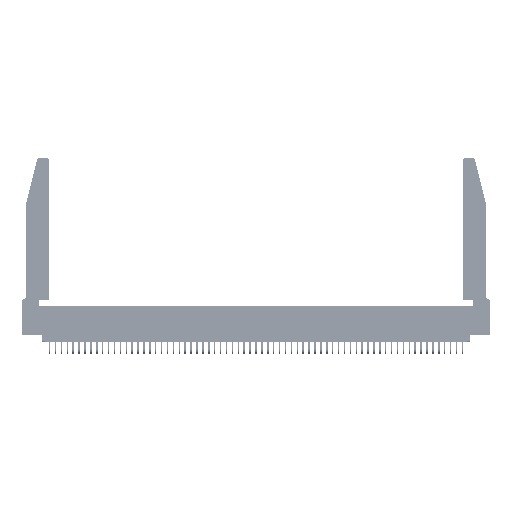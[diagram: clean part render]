
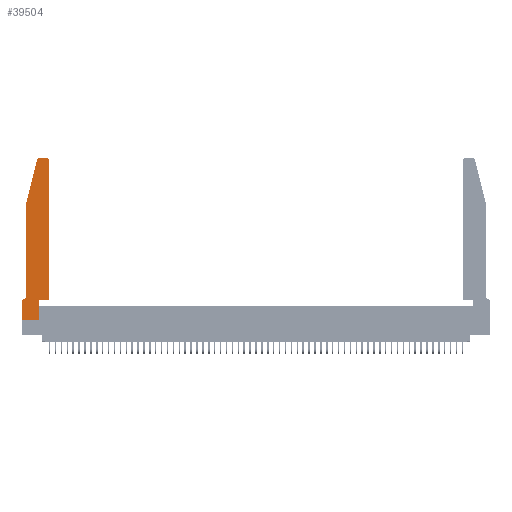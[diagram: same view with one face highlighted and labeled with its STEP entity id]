
A CAD part, top view. The second image highlights one B-rep face of the part: STEP entity #39504.
In plain terms, the highlighted planar face has unit normal (0, 0, 1).
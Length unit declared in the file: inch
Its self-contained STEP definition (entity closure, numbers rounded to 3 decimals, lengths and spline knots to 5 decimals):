
#1034 = VERTEX_POINT ( 'NONE', #20914 ) ;
#1150 = ORIENTED_EDGE ( 'NONE', *, *, #9812, .T. ) ;
#1171 = ORIENTED_EDGE ( 'NONE', *, *, #28467, .T. ) ;
#1255 = DIRECTION ( 'NONE',  ( 0., 0., 1. ) ) ;
#1803 = CARTESIAN_POINT ( 'NONE',  ( 0.25487, 2.72718, 0.37 ) ) ;
#3108 = ORIENTED_EDGE ( 'NONE', *, *, #34720, .T. ) ;
#3602 = VECTOR ( 'NONE', #41435, 39.37008 ) ;
#4488 = VECTOR ( 'NONE', #5732, 39.37008 ) ;
#5732 = DIRECTION ( 'NONE',  ( 0., -1., 0. ) ) ;
#5873 = VERTEX_POINT ( 'NONE', #36605 ) ;
#6295 = LINE ( 'NONE', #46896, #16879 ) ;
#6789 = CARTESIAN_POINT ( 'NONE',  ( 0.2865, 0., 0.37 ) ) ;
#7139 = DIRECTION ( 'NONE',  ( 0., 0., 1. ) ) ;
#7203 = VERTEX_POINT ( 'NONE', #6789 ) ;
#7731 = EDGE_LOOP ( 'NONE', ( #19353, #58043, #13046, #40859, #8081, #19368, #31691, #1150, #57109, #48052, #3108, #1171 ) ) ;
#8081 = ORIENTED_EDGE ( 'NONE', *, *, #39236, .T. ) ;
#9375 = DIRECTION ( 'NONE',  ( 0., 1., 0. ) ) ;
#9408 = VECTOR ( 'NONE', #23605, 39.37008 ) ;
#9812 = EDGE_CURVE ( 'NONE', #35734, #7203, #21348, .T. ) ;
#10364 = EDGE_CURVE ( 'NONE', #39100, #34004, #17067, .T. ) ;
#10908 = EDGE_CURVE ( 'NONE', #15181, #21581, #35340, .T. ) ;
#13046 = ORIENTED_EDGE ( 'NONE', *, *, #24477, .T. ) ;
#13069 = EDGE_CURVE ( 'NONE', #51149, #5873, #43283, .T. ) ;
#13524 = CARTESIAN_POINT ( 'NONE',  ( 0.284, 2.75, 0.37 ) ) ;
#15181 = VERTEX_POINT ( 'NONE', #21804 ) ;
#15740 = CARTESIAN_POINT ( 'NONE',  ( 0.4205, 2.72, 0.37 ) ) ;
#15949 = CARTESIAN_POINT ( 'NONE',  ( 0.2605, 2.75, 0.37 ) ) ;
#16007 = LINE ( 'NONE', #26669, #39957 ) ;
#16879 = VECTOR ( 'NONE', #33489, 39.37008 ) ;
#17067 = CIRCLE ( 'NONE', #20418, 0.03 ) ;
#17629 = DIRECTION ( 'NONE',  ( -0.239, -0.971, 0. ) ) ;
#19092 = CARTESIAN_POINT ( 'NONE',  ( 0., 0., 0.37 ) ) ;
#19340 = VECTOR ( 'NONE', #57221, 39.37008 ) ;
#19353 = ORIENTED_EDGE ( 'NONE', *, *, #34781, .T. ) ;
#19368 = ORIENTED_EDGE ( 'NONE', *, *, #13069, .T. ) ;
#20258 = DIRECTION ( 'NONE',  ( 1., 0., 0. ) ) ;
#20418 = AXIS2_PLACEMENT_3D ( 'NONE', #28280, #1255, #32839 ) ;
#20914 = CARTESIAN_POINT ( 'NONE',  ( 0.2865, 0.35, 0.37 ) ) ;
#21348 = LINE ( 'NONE', #19092, #9408 ) ;
#21581 = VERTEX_POINT ( 'NONE', #56674 ) ;
#21804 = CARTESIAN_POINT ( 'NONE',  ( 0.0755, 2., 0.37 ) ) ;
#21832 = DIRECTION ( 'NONE',  ( 1., 0., 0. ) ) ;
#22284 = VERTEX_POINT ( 'NONE', #38533 ) ;
#23109 = VECTOR ( 'NONE', #21832, 39.37008 ) ;
#23528 = DIRECTION ( 'NONE',  ( 0., 0., -1. ) ) ;
#23605 = DIRECTION ( 'NONE',  ( 1., 0., 0. ) ) ;
#24477 = EDGE_CURVE ( 'NONE', #34004, #15181, #16007, .T. ) ;
#24735 = AXIS2_PLACEMENT_3D ( 'NONE', #52037, #7139, #38683 ) ;
#25061 = PLANE ( 'NONE',  #24735 ) ;
#26669 = CARTESIAN_POINT ( 'NONE',  ( 0.0755, 2., 0.37 ) ) ;
#27659 = CARTESIAN_POINT ( 'NONE',  ( 0.4205, 2.75, 0.37 ) ) ;
#28280 = CARTESIAN_POINT ( 'NONE',  ( 0.284, 2.72, 0.37 ) ) ;
#28467 = EDGE_CURVE ( 'NONE', #37602, #40778, #28699, .T. ) ;
#28699 = CIRCLE ( 'NONE', #55699, 0.03 ) ;
#30979 = VECTOR ( 'NONE', #9375, 39.37008 ) ;
#31407 = CARTESIAN_POINT ( 'NONE',  ( 0., 0., 0.37 ) ) ;
#31691 = ORIENTED_EDGE ( 'NONE', *, *, #37896, .T. ) ;
#32839 = DIRECTION ( 'NONE',  ( 1., 0., 0. ) ) ;
#33489 = DIRECTION ( 'NONE',  ( 0., 1., 0. ) ) ;
#34004 = VERTEX_POINT ( 'NONE', #1803 ) ;
#34720 = EDGE_CURVE ( 'NONE', #22284, #37602, #6295, .T. ) ;
#34781 = EDGE_CURVE ( 'NONE', #40778, #39100, #38022, .T. ) ;
#35322 = CARTESIAN_POINT ( 'NONE',  ( 0.4505, 2.72, 0.37 ) ) ;
#35340 = LINE ( 'NONE', #36891, #3602 ) ;
#35734 = VERTEX_POINT ( 'NONE', #31407 ) ;
#36516 = LINE ( 'NONE', #44329, #23109 ) ;
#36605 = CARTESIAN_POINT ( 'NONE',  ( 0., 0.35, 0.37 ) ) ;
#36891 = CARTESIAN_POINT ( 'NONE',  ( 0.0755, 2., 0.37 ) ) ;
#37602 = VERTEX_POINT ( 'NONE', #35322 ) ;
#37896 = EDGE_CURVE ( 'NONE', #5873, #35734, #40470, .T. ) ;
#37986 = FACE_OUTER_BOUND ( 'NONE', #7731, .T. ) ;
#38022 = LINE ( 'NONE', #15949, #49990 ) ;
#38533 = CARTESIAN_POINT ( 'NONE',  ( 0.4505, 0.35, 0.37 ) ) ;
#38683 = DIRECTION ( 'NONE',  ( 1., 0., 0. ) ) ;
#39100 = VERTEX_POINT ( 'NONE', #13524 ) ;
#39160 = EDGE_CURVE ( 'NONE', #7203, #1034, #44385, .T. ) ;
#39236 = EDGE_CURVE ( 'NONE', #21581, #51149, #52077, .T. ) ;
#39504 = ADVANCED_FACE ( 'NONE', ( #37986 ), #25061, .T. ) ;
#39957 = VECTOR ( 'NONE', #17629, 39.37008 ) ;
#39962 = EDGE_CURVE ( 'NONE', #1034, #22284, #36516, .T. ) ;
#40470 = LINE ( 'NONE', #41616, #4488 ) ;
#40778 = VERTEX_POINT ( 'NONE', #27659 ) ;
#40859 = ORIENTED_EDGE ( 'NONE', *, *, #10908, .T. ) ;
#40993 = AXIS2_PLACEMENT_3D ( 'NONE', #50505, #23528, #55011 ) ;
#41435 = DIRECTION ( 'NONE',  ( 0., -1., 0. ) ) ;
#41616 = CARTESIAN_POINT ( 'NONE',  ( 0., 0., 0.37 ) ) ;
#43283 = LINE ( 'NONE', #52715, #19340 ) ;
#44329 = CARTESIAN_POINT ( 'NONE',  ( 0.4505, 0.35, 0.37 ) ) ;
#44385 = LINE ( 'NONE', #45425, #30979 ) ;
#45425 = CARTESIAN_POINT ( 'NONE',  ( 0.2865, 0.35, 0.37 ) ) ;
#46896 = CARTESIAN_POINT ( 'NONE',  ( 0.4505, 0.35, 0.37 ) ) ;
#47256 = DIRECTION ( 'NONE',  ( 0., 0., 1. ) ) ;
#47460 = DIRECTION ( 'NONE',  ( -1., 0., 0. ) ) ;
#48052 = ORIENTED_EDGE ( 'NONE', *, *, #39962, .T. ) ;
#49663 = CARTESIAN_POINT ( 'NONE',  ( 0.0055, 0.35, 0.37 ) ) ;
#49990 = VECTOR ( 'NONE', #47460, 39.37008 ) ;
#50505 = CARTESIAN_POINT ( 'NONE',  ( 0.0055, 0.42, 0.37 ) ) ;
#51149 = VERTEX_POINT ( 'NONE', #49663 ) ;
#52037 = CARTESIAN_POINT ( 'NONE',  ( 0., 0.35, 0.37 ) ) ;
#52077 = CIRCLE ( 'NONE', #40993, 0.07 ) ;
#52715 = CARTESIAN_POINT ( 'NONE',  ( 0.0755, 0.35, 0.37 ) ) ;
#55011 = DIRECTION ( 'NONE',  ( -1., 0., 0. ) ) ;
#55699 = AXIS2_PLACEMENT_3D ( 'NONE', #15740, #47256, #20258 ) ;
#56674 = CARTESIAN_POINT ( 'NONE',  ( 0.0755, 0.42, 0.37 ) ) ;
#57109 = ORIENTED_EDGE ( 'NONE', *, *, #39160, .T. ) ;
#57221 = DIRECTION ( 'NONE',  ( -1., 0., 0. ) ) ;
#58043 = ORIENTED_EDGE ( 'NONE', *, *, #10364, .T. ) ;
